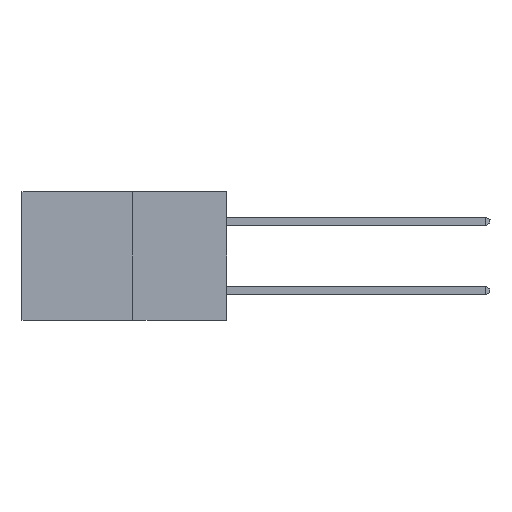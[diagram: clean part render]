
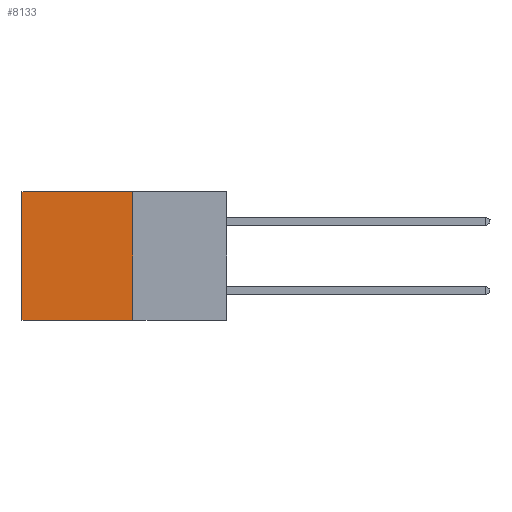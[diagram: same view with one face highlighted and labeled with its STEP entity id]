
A CAD part, left-side view. The second image highlights one B-rep face of the part: STEP entity #8133.
In plain terms, the highlighted planar face has unit normal (-1, 0, 0).
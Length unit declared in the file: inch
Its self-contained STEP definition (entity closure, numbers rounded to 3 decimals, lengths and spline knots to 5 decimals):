
#25 = LINE ( 'NONE', #6675, #3886 ) ;
#180 = DIRECTION ( 'NONE',  ( 0., 0., -1. ) ) ;
#600 = VECTOR ( 'NONE', #180, 39.37008 ) ;
#622 = CARTESIAN_POINT ( 'NONE',  ( 0.277, 0.27, -0.37 ) ) ;
#1031 = VERTEX_POINT ( 'NONE', #8136 ) ;
#1398 = DIRECTION ( 'NONE',  ( 0., 1., 0. ) ) ;
#1401 = LINE ( 'NONE', #6256, #8438 ) ;
#1507 = VECTOR ( 'NONE', #6521, 39.37008 ) ;
#1998 = EDGE_CURVE ( 'NONE', #1031, #3992, #3759, .T. ) ;
#2345 = ORIENTED_EDGE ( 'NONE', *, *, #7198, .T. ) ;
#2412 = CARTESIAN_POINT ( 'NONE',  ( 0.277, 0.59, -0.37 ) ) ;
#2596 = ORIENTED_EDGE ( 'NONE', *, *, #1998, .F. ) ;
#2714 = ORIENTED_EDGE ( 'NONE', *, *, #6076, .F. ) ;
#3100 = CARTESIAN_POINT ( 'NONE',  ( 0.277, 0.27, -0.37 ) ) ;
#3280 = ORIENTED_EDGE ( 'NONE', *, *, #4649, .T. ) ;
#3759 = LINE ( 'NONE', #6806, #1507 ) ;
#3886 = VECTOR ( 'NONE', #1398, 39.37008 ) ;
#3992 = VERTEX_POINT ( 'NONE', #3100 ) ;
#4176 = DIRECTION ( 'NONE',  ( 0., 1., 0. ) ) ;
#4421 = DIRECTION ( 'NONE',  ( 0., 0., -1. ) ) ;
#4528 = CARTESIAN_POINT ( 'NONE',  ( 0.277, 0.59, -0.37 ) ) ;
#4649 = EDGE_CURVE ( 'NONE', #1031, #7482, #1401, .T. ) ;
#5268 = CARTESIAN_POINT ( 'NONE',  ( 0.277, 0.59, 0. ) ) ;
#5706 = PLANE ( 'NONE',  #6103 ) ;
#6016 = EDGE_LOOP ( 'NONE', ( #2345, #2714, #2596, #3280 ) ) ;
#6076 = EDGE_CURVE ( 'NONE', #3992, #6207, #25, .T. ) ;
#6103 = AXIS2_PLACEMENT_3D ( 'NONE', #622, #8264, #4421 ) ;
#6121 = LINE ( 'NONE', #2412, #600 ) ;
#6207 = VERTEX_POINT ( 'NONE', #4528 ) ;
#6256 = CARTESIAN_POINT ( 'NONE',  ( 0.277, 0.27, 0. ) ) ;
#6521 = DIRECTION ( 'NONE',  ( 0., 0., -1. ) ) ;
#6675 = CARTESIAN_POINT ( 'NONE',  ( 0.277, 0.27, -0.37 ) ) ;
#6806 = CARTESIAN_POINT ( 'NONE',  ( 0.277, 0.27, -0.37 ) ) ;
#7198 = EDGE_CURVE ( 'NONE', #7482, #6207, #6121, .T. ) ;
#7482 = VERTEX_POINT ( 'NONE', #5268 ) ;
#8133 = ADVANCED_FACE ( 'NONE', ( #8199 ), #5706, .F. ) ;
#8136 = CARTESIAN_POINT ( 'NONE',  ( 0.277, 0.27, 0. ) ) ;
#8199 = FACE_OUTER_BOUND ( 'NONE', #6016, .T. ) ;
#8264 = DIRECTION ( 'NONE',  ( 1., 0., 0. ) ) ;
#8438 = VECTOR ( 'NONE', #4176, 39.37008 ) ;
